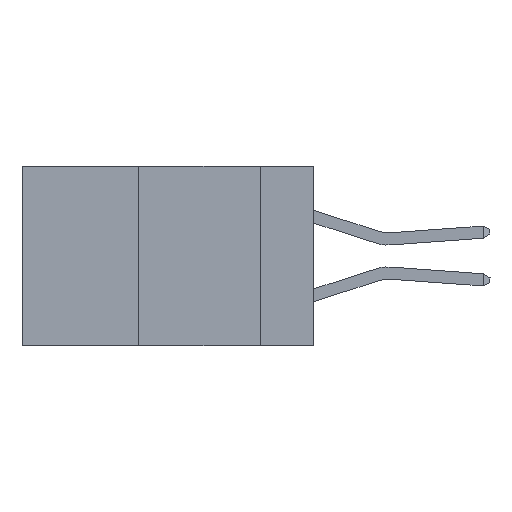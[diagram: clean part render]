
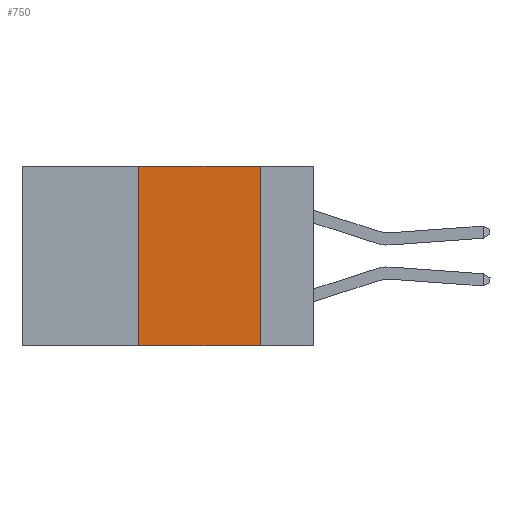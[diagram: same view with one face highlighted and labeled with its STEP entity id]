
A CAD part, left-side view. The second image highlights one B-rep face of the part: STEP entity #750.
In plain terms, the highlighted planar face has unit normal (-1, 0, 0).
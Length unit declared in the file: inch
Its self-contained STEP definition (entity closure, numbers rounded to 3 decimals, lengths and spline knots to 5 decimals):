
#88 = AXIS2_PLACEMENT_3D ( 'NONE', #11780, #11155, #11106 ) ;
#610 = EDGE_CURVE ( 'NONE', #10804, #20843, #15241, .T. ) ;
#750 = ADVANCED_FACE ( 'NONE', ( #12189 ), #12229, .F. ) ;
#883 = LINE ( 'NONE', #13655, #13854 ) ;
#2506 = EDGE_CURVE ( 'NONE', #18541, #10804, #9771, .T. ) ;
#5524 = LINE ( 'NONE', #11529, #9047 ) ;
#5734 = VECTOR ( 'NONE', #15415, 39.37008 ) ;
#6361 = VECTOR ( 'NONE', #11173, 39.37008 ) ;
#6625 = CARTESIAN_POINT ( 'NONE',  ( 0., 0.36, -0.37 ) ) ;
#7300 = VERTEX_POINT ( 'NONE', #6625 ) ;
#9047 = VECTOR ( 'NONE', #21177, 39.37008 ) ;
#9771 = LINE ( 'NONE', #12231, #5734 ) ;
#10457 = EDGE_LOOP ( 'NONE', ( #16063, #13040, #19414, #13585 ) ) ;
#10804 = VERTEX_POINT ( 'NONE', #17349 ) ;
#10826 = CARTESIAN_POINT ( 'NONE',  ( 0., 0.36, 0. ) ) ;
#10907 = CARTESIAN_POINT ( 'NONE',  ( 0., 0.11, 0. ) ) ;
#11106 = DIRECTION ( 'NONE',  ( 0., 0., -1. ) ) ;
#11155 = DIRECTION ( 'NONE',  ( 1., 0., 0. ) ) ;
#11173 = DIRECTION ( 'NONE',  ( 0., 0., -1. ) ) ;
#11529 = CARTESIAN_POINT ( 'NONE',  ( 0., 0.36, 0. ) ) ;
#11780 = CARTESIAN_POINT ( 'NONE',  ( 0., 0.6, 0. ) ) ;
#12189 = FACE_OUTER_BOUND ( 'NONE', #10457, .T. ) ;
#12229 = PLANE ( 'NONE',  #88 ) ;
#12231 = CARTESIAN_POINT ( 'NONE',  ( 0., 0.6, 0. ) ) ;
#12429 = EDGE_CURVE ( 'NONE', #7300, #18541, #5524, .T. ) ;
#13040 = ORIENTED_EDGE ( 'NONE', *, *, #2506, .F. ) ;
#13585 = ORIENTED_EDGE ( 'NONE', *, *, #16462, .T. ) ;
#13655 = CARTESIAN_POINT ( 'NONE',  ( 0., 0.6, -0.37 ) ) ;
#13854 = VECTOR ( 'NONE', #15338, 39.37008 ) ;
#15241 = LINE ( 'NONE', #10907, #6361 ) ;
#15338 = DIRECTION ( 'NONE',  ( 0., -1., 0. ) ) ;
#15415 = DIRECTION ( 'NONE',  ( 0., -1., 0. ) ) ;
#15897 = CARTESIAN_POINT ( 'NONE',  ( 0., 0.11, -0.37 ) ) ;
#16063 = ORIENTED_EDGE ( 'NONE', *, *, #610, .F. ) ;
#16462 = EDGE_CURVE ( 'NONE', #7300, #20843, #883, .T. ) ;
#17349 = CARTESIAN_POINT ( 'NONE',  ( 0., 0.11, 0. ) ) ;
#18541 = VERTEX_POINT ( 'NONE', #10826 ) ;
#19414 = ORIENTED_EDGE ( 'NONE', *, *, #12429, .F. ) ;
#20843 = VERTEX_POINT ( 'NONE', #15897 ) ;
#21177 = DIRECTION ( 'NONE',  ( 0., 0., 1. ) ) ;
